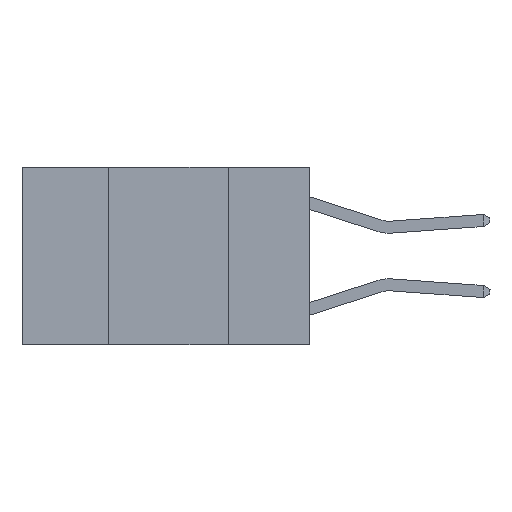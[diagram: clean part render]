
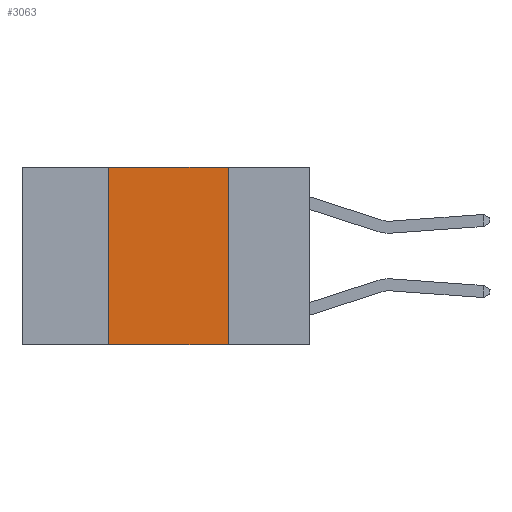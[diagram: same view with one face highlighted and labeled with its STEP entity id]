
A CAD part, left-side view. The second image highlights one B-rep face of the part: STEP entity #3063.
In plain terms, the highlighted planar face has unit normal (-1, 0, 0).
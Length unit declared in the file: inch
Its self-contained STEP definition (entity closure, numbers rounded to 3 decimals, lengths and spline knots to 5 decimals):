
#181 = VECTOR ( 'NONE', #1996, 39.37008 ) ;
#658 = CARTESIAN_POINT ( 'NONE',  ( 0., 0.6, 0. ) ) ;
#822 = CARTESIAN_POINT ( 'NONE',  ( 0., 0.17, -0.37 ) ) ;
#1408 = DIRECTION ( 'NONE',  ( 0., -1., 0. ) ) ;
#1887 = LINE ( 'NONE', #658, #5658 ) ;
#1996 = DIRECTION ( 'NONE',  ( 0., 0., 1. ) ) ;
#2256 = AXIS2_PLACEMENT_3D ( 'NONE', #8020, #2812, #3889 ) ;
#2812 = DIRECTION ( 'NONE',  ( 1., 0., 0. ) ) ;
#2901 = DIRECTION ( 'NONE',  ( 0., -1., 0. ) ) ;
#3063 = ADVANCED_FACE ( 'NONE', ( #8233 ), #8184, .F. ) ;
#3742 = VERTEX_POINT ( 'NONE', #9177 ) ;
#3889 = DIRECTION ( 'NONE',  ( 0., 0., -1. ) ) ;
#4152 = VERTEX_POINT ( 'NONE', #7094 ) ;
#4291 = LINE ( 'NONE', #6096, #181 ) ;
#4406 = LINE ( 'NONE', #7256, #5974 ) ;
#4461 = ORIENTED_EDGE ( 'NONE', *, *, #7969, .T. ) ;
#4627 = VECTOR ( 'NONE', #5033, 39.37008 ) ;
#4975 = CARTESIAN_POINT ( 'NONE',  ( 0., 0.17, 0. ) ) ;
#5033 = DIRECTION ( 'NONE',  ( 0., 0., -1. ) ) ;
#5352 = ORIENTED_EDGE ( 'NONE', *, *, #7066, .F. ) ;
#5658 = VECTOR ( 'NONE', #1408, 39.37008 ) ;
#5704 = VERTEX_POINT ( 'NONE', #4975 ) ;
#5974 = VECTOR ( 'NONE', #2901, 39.37008 ) ;
#6096 = CARTESIAN_POINT ( 'NONE',  ( 0., 0.42, 0. ) ) ;
#6516 = LINE ( 'NONE', #8561, #4627 ) ;
#6879 = EDGE_CURVE ( 'NONE', #3742, #5704, #1887, .T. ) ;
#7053 = VERTEX_POINT ( 'NONE', #822 ) ;
#7066 = EDGE_CURVE ( 'NONE', #4152, #3742, #4291, .T. ) ;
#7094 = CARTESIAN_POINT ( 'NONE',  ( 0., 0.42, -0.37 ) ) ;
#7256 = CARTESIAN_POINT ( 'NONE',  ( 0., 0.6, -0.37 ) ) ;
#7847 = EDGE_CURVE ( 'NONE', #5704, #7053, #6516, .T. ) ;
#7969 = EDGE_CURVE ( 'NONE', #4152, #7053, #4406, .T. ) ;
#8020 = CARTESIAN_POINT ( 'NONE',  ( 0., 0.6, 0. ) ) ;
#8184 = PLANE ( 'NONE',  #2256 ) ;
#8233 = FACE_OUTER_BOUND ( 'NONE', #8747, .T. ) ;
#8396 = ORIENTED_EDGE ( 'NONE', *, *, #7847, .F. ) ;
#8561 = CARTESIAN_POINT ( 'NONE',  ( 0., 0.17, 0. ) ) ;
#8658 = ORIENTED_EDGE ( 'NONE', *, *, #6879, .F. ) ;
#8747 = EDGE_LOOP ( 'NONE', ( #8396, #8658, #5352, #4461 ) ) ;
#9177 = CARTESIAN_POINT ( 'NONE',  ( 0., 0.42, 0. ) ) ;
